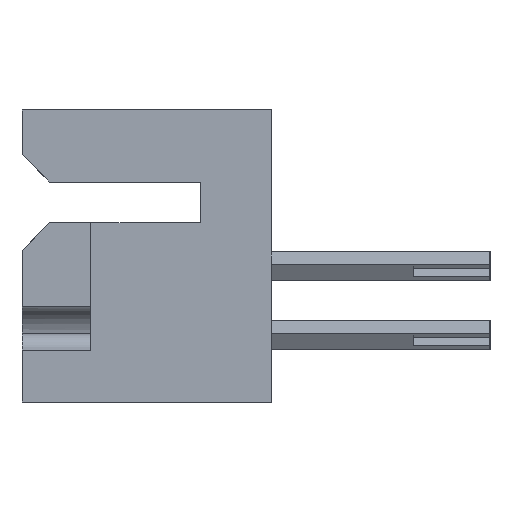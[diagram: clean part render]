
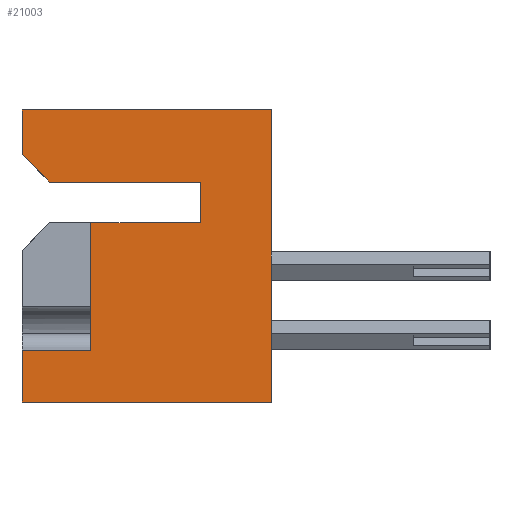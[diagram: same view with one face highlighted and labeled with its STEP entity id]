
A CAD part, left-side view. The second image highlights one B-rep face of the part: STEP entity #21003.
In plain terms, the highlighted planar face has unit normal (-1, 0, 0).
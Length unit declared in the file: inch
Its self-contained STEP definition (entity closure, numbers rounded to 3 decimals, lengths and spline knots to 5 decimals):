
#188 = EDGE_CURVE ( 'NONE', #4670, #12889, #8402, .T. ) ;
#831 = VECTOR ( 'NONE', #11962, 39.37008 ) ;
#1893 = VERTEX_POINT ( 'NONE', #4096 ) ;
#2330 = CARTESIAN_POINT ( 'NONE',  ( 0., 0.453, 0. ) ) ;
#2344 = EDGE_CURVE ( 'NONE', #16494, #6276, #16675, .T. ) ;
#4096 = CARTESIAN_POINT ( 'NONE',  ( 0., 0.453, -0.437 ) ) ;
#4489 = ORIENTED_EDGE ( 'NONE', *, *, #25040, .F. ) ;
#4522 = CARTESIAN_POINT ( 'NONE',  ( 0., 0.328, -0.437 ) ) ;
#4609 = VECTOR ( 'NONE', #20786, 39.37008 ) ;
#4670 = VERTEX_POINT ( 'NONE', #4848 ) ;
#4848 = CARTESIAN_POINT ( 'NONE',  ( 0., 0.453, -0.531 ) ) ;
#4948 = VERTEX_POINT ( 'NONE', #22787 ) ;
#5290 = CARTESIAN_POINT ( 'NONE',  ( 0., 0.453, 0. ) ) ;
#5802 = FACE_OUTER_BOUND ( 'NONE', #14067, .T. ) ;
#6052 = VECTOR ( 'NONE', #18979, 39.37008 ) ;
#6276 = VERTEX_POINT ( 'NONE', #25419 ) ;
#6568 = AXIS2_PLACEMENT_3D ( 'NONE', #15052, #17099, #17401 ) ;
#7666 = VECTOR ( 'NONE', #20323, 39.37008 ) ;
#7917 = PLANE ( 'NONE',  #6568 ) ;
#8022 = VERTEX_POINT ( 'NONE', #4522 ) ;
#8092 = DIRECTION ( 'NONE',  ( 0., 0., 1. ) ) ;
#8323 = DIRECTION ( 'NONE',  ( 0., 0., 1. ) ) ;
#8402 = LINE ( 'NONE', #26933, #7666 ) ;
#8977 = DIRECTION ( 'NONE',  ( 0., 1., 0. ) ) ;
#8990 = EDGE_CURVE ( 'NONE', #15266, #6276, #11762, .T. ) ;
#9232 = ORIENTED_EDGE ( 'NONE', *, *, #29697, .F. ) ;
#9536 = VECTOR ( 'NONE', #10440, 39.37008 ) ;
#9870 = LINE ( 'NONE', #29339, #15773 ) ;
#9966 = EDGE_CURVE ( 'NONE', #23557, #4948, #9870, .T. ) ;
#9996 = ORIENTED_EDGE ( 'NONE', *, *, #17527, .F. ) ;
#10440 = DIRECTION ( 'NONE',  ( 0., -0.707, -0.707 ) ) ;
#10907 = CARTESIAN_POINT ( 'NONE',  ( 0., 0.128, -0.205 ) ) ;
#10913 = ORIENTED_EDGE ( 'NONE', *, *, #30640, .T. ) ;
#11279 = CARTESIAN_POINT ( 'NONE',  ( 0., 0.128, -0.131 ) ) ;
#11660 = EDGE_CURVE ( 'NONE', #8022, #4948, #13093, .T. ) ;
#11670 = LINE ( 'NONE', #2330, #4609 ) ;
#11762 = LINE ( 'NONE', #27375, #9536 ) ;
#11962 = DIRECTION ( 'NONE',  ( 0., 0., 1. ) ) ;
#12889 = VERTEX_POINT ( 'NONE', #20961 ) ;
#12946 = VECTOR ( 'NONE', #21468, 39.37008 ) ;
#13093 = LINE ( 'NONE', #27125, #18613 ) ;
#13463 = LINE ( 'NONE', #21264, #831 ) ;
#13497 = CARTESIAN_POINT ( 'NONE',  ( 0., 0.328, -0.437 ) ) ;
#13610 = CARTESIAN_POINT ( 'NONE',  ( 0., 0.128, -0.131 ) ) ;
#14067 = EDGE_LOOP ( 'NONE', ( #10913, #9232, #21565, #19379, #9996, #4489, #16811, #14078, #21449, #19426, #25544 ) ) ;
#14078 = ORIENTED_EDGE ( 'NONE', *, *, #2344, .F. ) ;
#14234 = CARTESIAN_POINT ( 'NONE',  ( 0., 0.128, -0.131 ) ) ;
#15052 = CARTESIAN_POINT ( 'NONE',  ( 0., 0.453, 0. ) ) ;
#15266 = VERTEX_POINT ( 'NONE', #25210 ) ;
#15773 = VECTOR ( 'NONE', #29133, 39.37008 ) ;
#16151 = LINE ( 'NONE', #13497, #29560 ) ;
#16494 = VERTEX_POINT ( 'NONE', #11279 ) ;
#16675 = LINE ( 'NONE', #13610, #29359 ) ;
#16811 = ORIENTED_EDGE ( 'NONE', *, *, #8990, .T. ) ;
#17099 = DIRECTION ( 'NONE',  ( 1., 0., 0. ) ) ;
#17401 = DIRECTION ( 'NONE',  ( 0., 0., -1. ) ) ;
#17527 = EDGE_CURVE ( 'NONE', #20906, #27256, #28187, .T. ) ;
#17668 = LINE ( 'NONE', #19862, #28141 ) ;
#18440 = DIRECTION ( 'NONE',  ( 0., 1., 0. ) ) ;
#18613 = VECTOR ( 'NONE', #8323, 39.37008 ) ;
#18979 = DIRECTION ( 'NONE',  ( 0., 0., 1. ) ) ;
#19379 = ORIENTED_EDGE ( 'NONE', *, *, #25673, .T. ) ;
#19426 = ORIENTED_EDGE ( 'NONE', *, *, #9966, .T. ) ;
#19862 = CARTESIAN_POINT ( 'NONE',  ( 0., 0.453, 0. ) ) ;
#20323 = DIRECTION ( 'NONE',  ( 0., -1., 0. ) ) ;
#20786 = DIRECTION ( 'NONE',  ( 0., 0., 1. ) ) ;
#20906 = VERTEX_POINT ( 'NONE', #24091 ) ;
#20961 = CARTESIAN_POINT ( 'NONE',  ( 0., 0., -0.531 ) ) ;
#21003 = ADVANCED_FACE ( 'NONE', ( #5802 ), #7917, .F. ) ;
#21264 = CARTESIAN_POINT ( 'NONE',  ( 0., 0., 0. ) ) ;
#21449 = ORIENTED_EDGE ( 'NONE', *, *, #25717, .F. ) ;
#21468 = DIRECTION ( 'NONE',  ( 0., -1., 0. ) ) ;
#21565 = ORIENTED_EDGE ( 'NONE', *, *, #188, .T. ) ;
#22787 = CARTESIAN_POINT ( 'NONE',  ( 0., 0.328, -0.205 ) ) ;
#23557 = VERTEX_POINT ( 'NONE', #10907 ) ;
#24091 = CARTESIAN_POINT ( 'NONE',  ( 0., 0.453, 0. ) ) ;
#25040 = EDGE_CURVE ( 'NONE', #15266, #20906, #11670, .T. ) ;
#25210 = CARTESIAN_POINT ( 'NONE',  ( 0., 0.453, -0.081 ) ) ;
#25419 = CARTESIAN_POINT ( 'NONE',  ( 0., 0.403, -0.131 ) ) ;
#25544 = ORIENTED_EDGE ( 'NONE', *, *, #11660, .F. ) ;
#25673 = EDGE_CURVE ( 'NONE', #12889, #27256, #13463, .T. ) ;
#25717 = EDGE_CURVE ( 'NONE', #23557, #16494, #29125, .T. ) ;
#26933 = CARTESIAN_POINT ( 'NONE',  ( 0., 0.453, -0.531 ) ) ;
#27125 = CARTESIAN_POINT ( 'NONE',  ( 0., 0.328, -0.205 ) ) ;
#27256 = VERTEX_POINT ( 'NONE', #27910 ) ;
#27375 = CARTESIAN_POINT ( 'NONE',  ( 0., 0.403, -0.131 ) ) ;
#27910 = CARTESIAN_POINT ( 'NONE',  ( 0., 0., 0. ) ) ;
#28141 = VECTOR ( 'NONE', #8092, 39.37008 ) ;
#28187 = LINE ( 'NONE', #5290, #12946 ) ;
#29125 = LINE ( 'NONE', #14234, #6052 ) ;
#29133 = DIRECTION ( 'NONE',  ( 0., 1., 0. ) ) ;
#29339 = CARTESIAN_POINT ( 'NONE',  ( 0., 0.128, -0.205 ) ) ;
#29359 = VECTOR ( 'NONE', #8977, 39.37008 ) ;
#29560 = VECTOR ( 'NONE', #18440, 39.37008 ) ;
#29697 = EDGE_CURVE ( 'NONE', #4670, #1893, #17668, .T. ) ;
#30640 = EDGE_CURVE ( 'NONE', #8022, #1893, #16151, .T. ) ;
